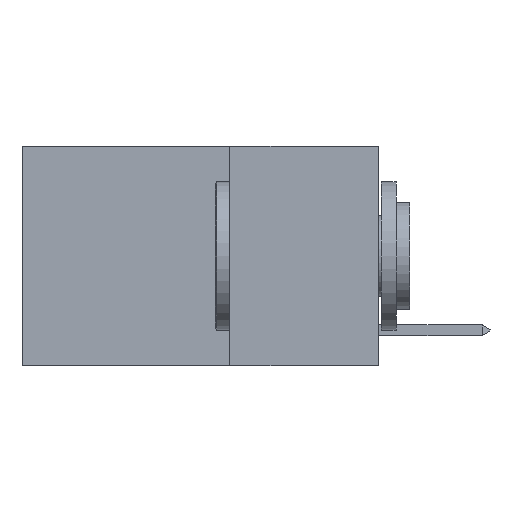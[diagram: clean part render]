
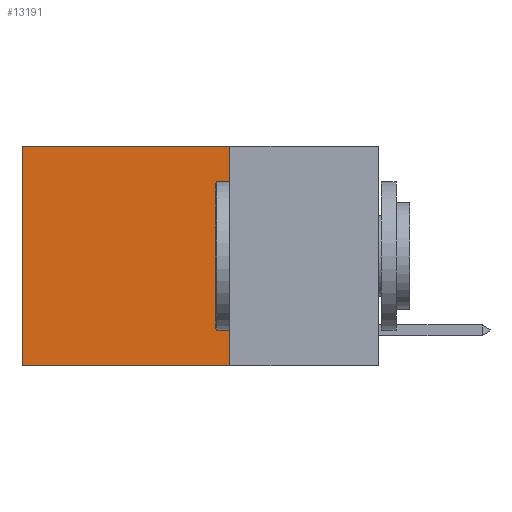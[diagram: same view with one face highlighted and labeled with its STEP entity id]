
A CAD part, left-side view. The second image highlights one B-rep face of the part: STEP entity #13191.
In plain terms, the highlighted planar face has unit normal (-1, 0, 0).
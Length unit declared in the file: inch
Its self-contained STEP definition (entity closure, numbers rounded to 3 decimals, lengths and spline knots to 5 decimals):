
#518 = EDGE_CURVE ( 'NONE', #16780, #557, #1762, .T. ) ;
#557 = VERTEX_POINT ( 'NONE', #2814 ) ;
#1033 = CARTESIAN_POINT ( 'NONE',  ( 0.2625, 0.25, 0. ) ) ;
#1470 = CARTESIAN_POINT ( 'NONE',  ( 0.2625, 0.25, 0. ) ) ;
#1762 = LINE ( 'NONE', #4164, #12193 ) ;
#2541 = CARTESIAN_POINT ( 'NONE',  ( 0.2625, 0.25, -0.37 ) ) ;
#2799 = LINE ( 'NONE', #1033, #7014 ) ;
#2814 = CARTESIAN_POINT ( 'NONE',  ( 0.2625, 0.6, -0.37 ) ) ;
#3281 = CARTESIAN_POINT ( 'NONE',  ( 0.2625, 0.25, 0. ) ) ;
#3573 = EDGE_CURVE ( 'NONE', #16093, #10237, #2799, .T. ) ;
#4139 = DIRECTION ( 'NONE',  ( 0., 1., 0. ) ) ;
#4164 = CARTESIAN_POINT ( 'NONE',  ( 0.2625, 0.25, -0.37 ) ) ;
#4597 = EDGE_LOOP ( 'NONE', ( #25795, #25113, #25559, #11170 ) ) ;
#5664 = DIRECTION ( 'NONE',  ( 0., 0., -1. ) ) ;
#6031 = LINE ( 'NONE', #3281, #21933 ) ;
#7014 = VECTOR ( 'NONE', #15634, 39.37008 ) ;
#8135 = CARTESIAN_POINT ( 'NONE',  ( 0.2625, 0.6, 0. ) ) ;
#10237 = VERTEX_POINT ( 'NONE', #8135 ) ;
#11170 = ORIENTED_EDGE ( 'NONE', *, *, #3573, .T. ) ;
#12193 = VECTOR ( 'NONE', #4139, 39.37008 ) ;
#12789 = CARTESIAN_POINT ( 'NONE',  ( 0.2625, 0.25, 0. ) ) ;
#13191 = ADVANCED_FACE ( 'NONE', ( #15971 ), #13989, .F. ) ;
#13989 = PLANE ( 'NONE',  #14988 ) ;
#14988 = AXIS2_PLACEMENT_3D ( 'NONE', #1470, #18119, #5664 ) ;
#15634 = DIRECTION ( 'NONE',  ( 0., 1., 0. ) ) ;
#15971 = FACE_OUTER_BOUND ( 'NONE', #4597, .T. ) ;
#16093 = VERTEX_POINT ( 'NONE', #12789 ) ;
#16780 = VERTEX_POINT ( 'NONE', #2541 ) ;
#17282 = LINE ( 'NONE', #19617, #23297 ) ;
#18119 = DIRECTION ( 'NONE',  ( 1., 0., 0. ) ) ;
#18195 = EDGE_CURVE ( 'NONE', #16093, #16780, #6031, .T. ) ;
#19617 = CARTESIAN_POINT ( 'NONE',  ( 0.2625, 0.6, 0. ) ) ;
#19910 = DIRECTION ( 'NONE',  ( 0., 0., -1. ) ) ;
#21657 = DIRECTION ( 'NONE',  ( 0., 0., -1. ) ) ;
#21933 = VECTOR ( 'NONE', #19910, 39.37008 ) ;
#23297 = VECTOR ( 'NONE', #21657, 39.37008 ) ;
#24056 = EDGE_CURVE ( 'NONE', #10237, #557, #17282, .T. ) ;
#25113 = ORIENTED_EDGE ( 'NONE', *, *, #518, .F. ) ;
#25559 = ORIENTED_EDGE ( 'NONE', *, *, #18195, .F. ) ;
#25795 = ORIENTED_EDGE ( 'NONE', *, *, #24056, .T. ) ;
